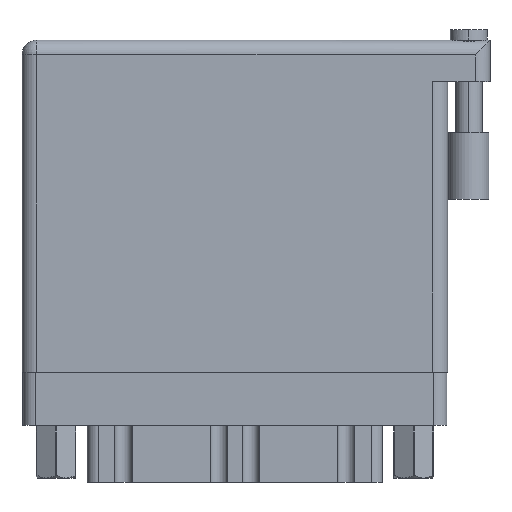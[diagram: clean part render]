
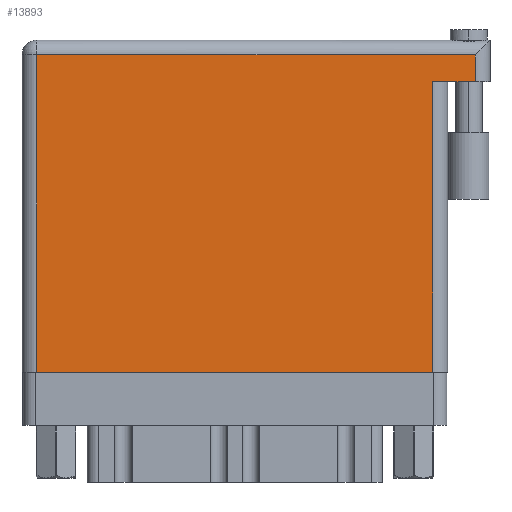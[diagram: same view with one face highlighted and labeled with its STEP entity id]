
A CAD part, front view. The second image highlights one B-rep face of the part: STEP entity #13893.
In plain terms, the highlighted face is planar.
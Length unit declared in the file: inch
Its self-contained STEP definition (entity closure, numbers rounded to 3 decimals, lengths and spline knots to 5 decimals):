
#383 = CARTESIAN_POINT ( 'NONE',  ( 0.07, 0., 0. ) ) ;
#471 = VECTOR ( 'NONE', #35166, 39.37008 ) ;
#5397 = CARTESIAN_POINT ( 'NONE',  ( 2.138, 1.369, 0. ) ) ;
#6133 = VERTEX_POINT ( 'NONE', #38407 ) ;
#6629 = VECTOR ( 'NONE', #21046, 39.37008 ) ;
#7101 = CARTESIAN_POINT ( 'NONE',  ( 2.138, 1.496, 0. ) ) ;
#7223 = DIRECTION ( 'NONE',  ( -1., 0., 0. ) ) ;
#8923 = CARTESIAN_POINT ( 'NONE',  ( 1.938, 1.369, 0. ) ) ;
#9484 = EDGE_CURVE ( 'NONE', #18527, #6133, #11656, .T. ) ;
#9838 = ORIENTED_EDGE ( 'NONE', *, *, #37678, .F. ) ;
#10585 = VECTOR ( 'NONE', #20400, 39.37008 ) ;
#11260 = LINE ( 'NONE', #28970, #14382 ) ;
#11552 = VECTOR ( 'NONE', #40521, 39.37008 ) ;
#11656 = LINE ( 'NONE', #33380, #11552 ) ;
#13823 = ORIENTED_EDGE ( 'NONE', *, *, #9484, .T. ) ;
#13893 = ADVANCED_FACE ( 'NONE', ( #15325 ), #29898, .F. ) ;
#14382 = VECTOR ( 'NONE', #15084, 39.37008 ) ;
#15084 = DIRECTION ( 'NONE',  ( -1., 0., 0. ) ) ;
#15325 = FACE_OUTER_BOUND ( 'NONE', #18124, .T. ) ;
#16264 = CARTESIAN_POINT ( 'NONE',  ( 0.07, 1.496, 0. ) ) ;
#17114 = AXIS2_PLACEMENT_3D ( 'NONE', #21793, #22734, #7223 ) ;
#18124 = EDGE_LOOP ( 'NONE', ( #13823, #37769, #9838, #33231, #34889, #37459 ) ) ;
#18527 = VERTEX_POINT ( 'NONE', #383 ) ;
#18794 = EDGE_CURVE ( 'NONE', #23484, #18527, #46828, .T. ) ;
#20400 = DIRECTION ( 'NONE',  ( 0., 1., 0. ) ) ;
#21046 = DIRECTION ( 'NONE',  ( 0., 1., 0. ) ) ;
#21793 = CARTESIAN_POINT ( 'NONE',  ( 0., 1.566, 0. ) ) ;
#22734 = DIRECTION ( 'NONE',  ( 0., 0., -1. ) ) ;
#23484 = VERTEX_POINT ( 'NONE', #16264 ) ;
#24386 = LINE ( 'NONE', #28445, #6629 ) ;
#25745 = CARTESIAN_POINT ( 'NONE',  ( 0., 1.496, 0. ) ) ;
#25815 = VECTOR ( 'NONE', #35964, 39.37008 ) ;
#28445 = CARTESIAN_POINT ( 'NONE',  ( 2.138, 1.566, 0. ) ) ;
#28970 = CARTESIAN_POINT ( 'NONE',  ( 2.208, 1.369, 0. ) ) ;
#29898 = PLANE ( 'NONE',  #17114 ) ;
#31837 = LINE ( 'NONE', #38510, #10585 ) ;
#33231 = ORIENTED_EDGE ( 'NONE', *, *, #36423, .T. ) ;
#33380 = CARTESIAN_POINT ( 'NONE',  ( 0., 0., 0. ) ) ;
#34889 = ORIENTED_EDGE ( 'NONE', *, *, #37120, .T. ) ;
#35166 = DIRECTION ( 'NONE',  ( 0., -1., 0. ) ) ;
#35410 = CARTESIAN_POINT ( 'NONE',  ( 0.07, 0., 0. ) ) ;
#35964 = DIRECTION ( 'NONE',  ( -1., 0., 0. ) ) ;
#36423 = EDGE_CURVE ( 'NONE', #42798, #38527, #24386, .T. ) ;
#37120 = EDGE_CURVE ( 'NONE', #38527, #23484, #43826, .T. ) ;
#37459 = ORIENTED_EDGE ( 'NONE', *, *, #18794, .T. ) ;
#37678 = EDGE_CURVE ( 'NONE', #42798, #46741, #11260, .T. ) ;
#37769 = ORIENTED_EDGE ( 'NONE', *, *, #40053, .T. ) ;
#38407 = CARTESIAN_POINT ( 'NONE',  ( 1.938, 0., 0. ) ) ;
#38510 = CARTESIAN_POINT ( 'NONE',  ( 1.938, 1.369, 0. ) ) ;
#38527 = VERTEX_POINT ( 'NONE', #7101 ) ;
#40053 = EDGE_CURVE ( 'NONE', #6133, #46741, #31837, .T. ) ;
#40521 = DIRECTION ( 'NONE',  ( 1., 0., 0. ) ) ;
#42798 = VERTEX_POINT ( 'NONE', #5397 ) ;
#43826 = LINE ( 'NONE', #25745, #25815 ) ;
#46741 = VERTEX_POINT ( 'NONE', #8923 ) ;
#46828 = LINE ( 'NONE', #35410, #471 ) ;
